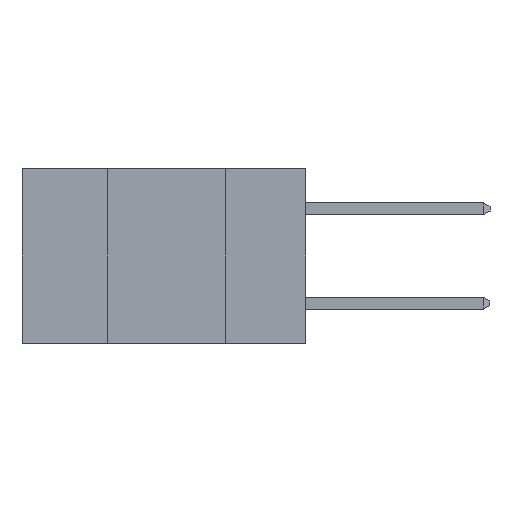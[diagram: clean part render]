
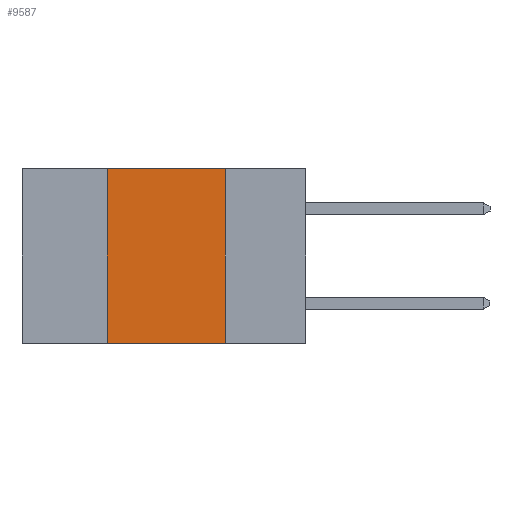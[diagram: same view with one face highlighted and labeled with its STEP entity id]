
A CAD part, left-side view. The second image highlights one B-rep face of the part: STEP entity #9587.
In plain terms, the highlighted planar face has unit normal (-1, 0, 0).
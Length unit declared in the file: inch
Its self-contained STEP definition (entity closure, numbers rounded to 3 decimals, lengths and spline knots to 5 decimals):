
#1655 = LINE ( 'NONE', #23167, #20808 ) ;
#2364 = VERTEX_POINT ( 'NONE', #2715 ) ;
#2467 = EDGE_CURVE ( 'NONE', #8905, #2364, #13400, .T. ) ;
#2567 = CARTESIAN_POINT ( 'NONE',  ( 0., 0.42, 0. ) ) ;
#2715 = CARTESIAN_POINT ( 'NONE',  ( 0., 0.17, 0. ) ) ;
#4138 = DIRECTION ( 'NONE',  ( 0., 0., 1. ) ) ;
#4681 = CARTESIAN_POINT ( 'NONE',  ( 0., 0.6, -0.37 ) ) ;
#6490 = VECTOR ( 'NONE', #9260, 39.37008 ) ;
#6566 = FACE_OUTER_BOUND ( 'NONE', #28682, .T. ) ;
#8029 = CARTESIAN_POINT ( 'NONE',  ( 0., 0.42, -0.37 ) ) ;
#8905 = VERTEX_POINT ( 'NONE', #2567 ) ;
#9260 = DIRECTION ( 'NONE',  ( 0., 0., -1. ) ) ;
#9513 = DIRECTION ( 'NONE',  ( 0., -1., 0. ) ) ;
#9587 = ADVANCED_FACE ( 'NONE', ( #6566 ), #11165, .F. ) ;
#11165 = PLANE ( 'NONE',  #17050 ) ;
#11352 = LINE ( 'NONE', #23544, #6490 ) ;
#12548 = VERTEX_POINT ( 'NONE', #24374 ) ;
#12674 = VECTOR ( 'NONE', #30429, 39.37008 ) ;
#13400 = LINE ( 'NONE', #13744, #12674 ) ;
#13744 = CARTESIAN_POINT ( 'NONE',  ( 0., 0.6, 0. ) ) ;
#15891 = EDGE_CURVE ( 'NONE', #2364, #12548, #11352, .T. ) ;
#15996 = DIRECTION ( 'NONE',  ( 0., 0., -1. ) ) ;
#16910 = VERTEX_POINT ( 'NONE', #8029 ) ;
#17050 = AXIS2_PLACEMENT_3D ( 'NONE', #27746, #30073, #15996 ) ;
#19135 = ORIENTED_EDGE ( 'NONE', *, *, #15891, .F. ) ;
#20135 = ORIENTED_EDGE ( 'NONE', *, *, #2467, .F. ) ;
#20390 = ORIENTED_EDGE ( 'NONE', *, *, #23866, .F. ) ;
#20808 = VECTOR ( 'NONE', #4138, 39.37008 ) ;
#21318 = ORIENTED_EDGE ( 'NONE', *, *, #21706, .T. ) ;
#21706 = EDGE_CURVE ( 'NONE', #16910, #12548, #29842, .T. ) ;
#23167 = CARTESIAN_POINT ( 'NONE',  ( 0., 0.42, 0. ) ) ;
#23544 = CARTESIAN_POINT ( 'NONE',  ( 0., 0.17, 0. ) ) ;
#23696 = VECTOR ( 'NONE', #9513, 39.37008 ) ;
#23866 = EDGE_CURVE ( 'NONE', #16910, #8905, #1655, .T. ) ;
#24374 = CARTESIAN_POINT ( 'NONE',  ( 0., 0.17, -0.37 ) ) ;
#27746 = CARTESIAN_POINT ( 'NONE',  ( 0., 0.6, 0. ) ) ;
#28682 = EDGE_LOOP ( 'NONE', ( #19135, #20135, #20390, #21318 ) ) ;
#29842 = LINE ( 'NONE', #4681, #23696 ) ;
#30073 = DIRECTION ( 'NONE',  ( 1., 0., 0. ) ) ;
#30429 = DIRECTION ( 'NONE',  ( 0., -1., 0. ) ) ;
